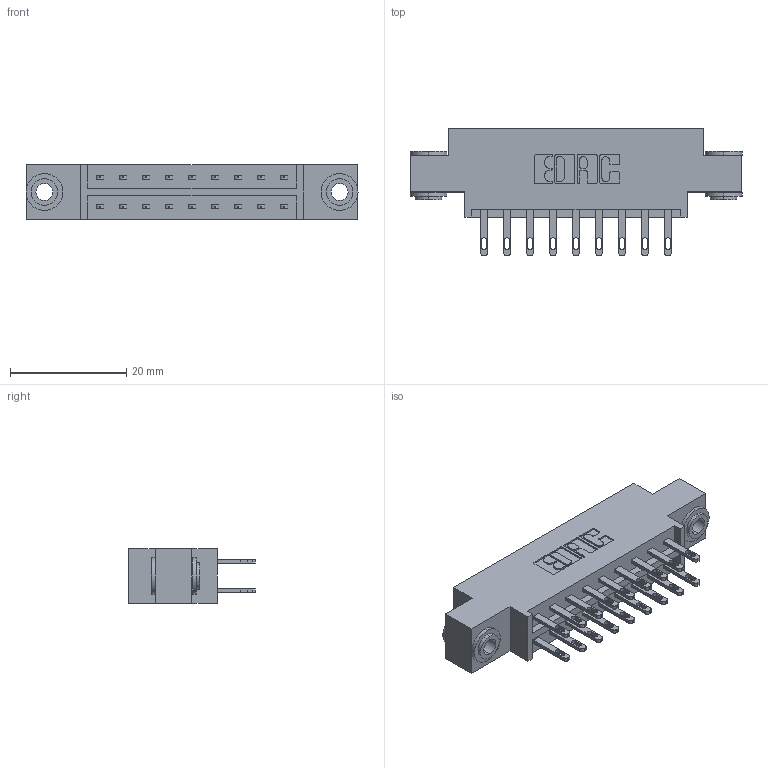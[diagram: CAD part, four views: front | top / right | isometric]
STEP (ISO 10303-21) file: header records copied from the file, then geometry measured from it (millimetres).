
FILE_DESCRIPTION (( 'STEP AP203' ), '1' );
FILE_NAME ('333-018-500-803.STEP', '2019-08-09T12:35:15', ( '' ), ( '' ), 'SwSTEP 2.0', 'SolidWorks 2016', '' );
FILE_SCHEMA (( 'CONFIG_CONTROL_DESIGN' ));
Length unit declared in the file: inch
Products named in the file (4): 345-292-001_345-293-100; 345-250-002_345-250-002-102; 333-018-500-803; 333 Part_Offset - .156 Dia - TH
Assembly tree (21 placements, depth 2):
  333-018-500-803
    333 Part_Offset - .156 Dia - TH
    345-292-001_345-293-100  x18
    345-250-002_345-250-002-102  x2
Bounding box: 57.2 x 21.85 x 9.4 mm (x, y, z)
Volume: 5377.9 mm3; surface area: 6643.2 mm2
Topology: 21 solids, 21 shells, 1020 faces, 3045 edges, 2026 vertices
Faces by surface type: plane 624, cylinder 388, cone 8
Entity records: 10770 total; most frequent: CARTESIAN_POINT 1801, ORIENTED_EDGE 1730, DIRECTION 1631, EDGE_CURVE 865, LINE 709, VECTOR 709, VERTEX_POINT 574, AXIS2_PLACEMENT_3D 461
